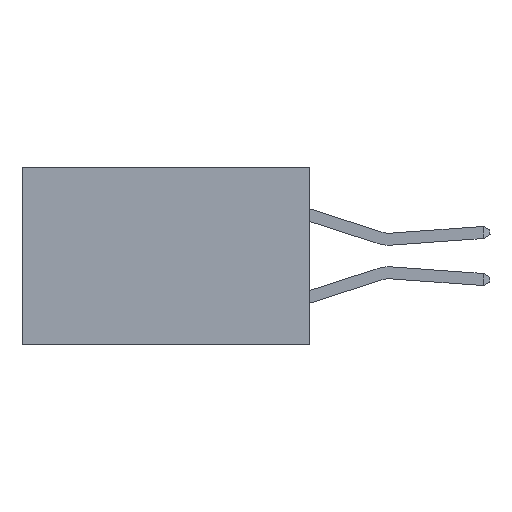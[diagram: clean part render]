
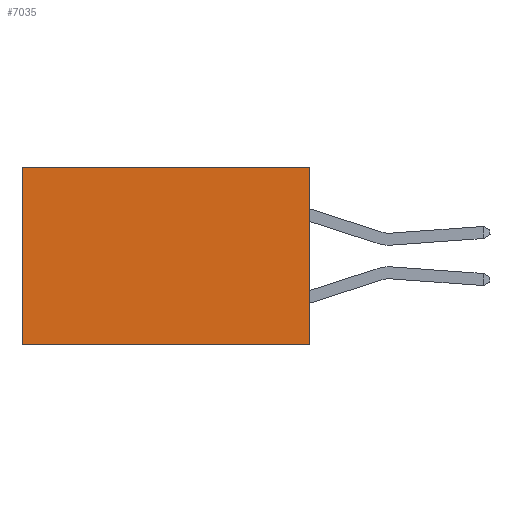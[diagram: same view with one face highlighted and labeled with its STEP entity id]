
A CAD part, left-side view. The second image highlights one B-rep face of the part: STEP entity #7035.
In plain terms, the highlighted planar face has unit normal (-1, 0, 0).
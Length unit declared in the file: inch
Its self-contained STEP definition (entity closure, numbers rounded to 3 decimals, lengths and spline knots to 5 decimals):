
#592 = CARTESIAN_POINT ( 'NONE',  ( 0.2615, 0., 0. ) ) ;
#673 = DIRECTION ( 'NONE',  ( 1., 0., 0. ) ) ;
#1024 = EDGE_CURVE ( 'NONE', #16479, #13670, #17530, .T. ) ;
#1749 = CARTESIAN_POINT ( 'NONE',  ( 0.2615, 0., -0.37 ) ) ;
#1981 = DIRECTION ( 'NONE',  ( 0., 0., -1. ) ) ;
#4610 = DIRECTION ( 'NONE',  ( 0., 0., -1. ) ) ;
#5098 = ORIENTED_EDGE ( 'NONE', *, *, #10494, .F. ) ;
#6005 = PLANE ( 'NONE',  #18022 ) ;
#7035 = ADVANCED_FACE ( 'NONE', ( #8070 ), #6005, .F. ) ;
#7647 = DIRECTION ( 'NONE',  ( 0., 1., 0. ) ) ;
#7846 = LINE ( 'NONE', #9695, #20229 ) ;
#8070 = FACE_OUTER_BOUND ( 'NONE', #13465, .T. ) ;
#8399 = CARTESIAN_POINT ( 'NONE',  ( 0.2615, 0.6, 0. ) ) ;
#9695 = CARTESIAN_POINT ( 'NONE',  ( 0.2615, 0., -0.37 ) ) ;
#9732 = ORIENTED_EDGE ( 'NONE', *, *, #21567, .T. ) ;
#9809 = CARTESIAN_POINT ( 'NONE',  ( 0.2615, 0., -0.37 ) ) ;
#10273 = CARTESIAN_POINT ( 'NONE',  ( 0.2615, 0., 0. ) ) ;
#10494 = EDGE_CURVE ( 'NONE', #13670, #15397, #7846, .T. ) ;
#11269 = EDGE_CURVE ( 'NONE', #16479, #18366, #18108, .T. ) ;
#13465 = EDGE_LOOP ( 'NONE', ( #9732, #5098, #20889, #18649 ) ) ;
#13670 = VERTEX_POINT ( 'NONE', #14851 ) ;
#13693 = VECTOR ( 'NONE', #1981, 39.37008 ) ;
#14851 = CARTESIAN_POINT ( 'NONE',  ( 0.2615, 0., -0.37 ) ) ;
#15397 = VERTEX_POINT ( 'NONE', #22271 ) ;
#15746 = VECTOR ( 'NONE', #4610, 39.37008 ) ;
#16479 = VERTEX_POINT ( 'NONE', #10273 ) ;
#16928 = CARTESIAN_POINT ( 'NONE',  ( 0.2615, 0.6, -0.37 ) ) ;
#16980 = VECTOR ( 'NONE', #7647, 39.37008 ) ;
#17530 = LINE ( 'NONE', #1749, #13693 ) ;
#18022 = AXIS2_PLACEMENT_3D ( 'NONE', #9809, #673, #20157 ) ;
#18108 = LINE ( 'NONE', #592, #16980 ) ;
#18366 = VERTEX_POINT ( 'NONE', #8399 ) ;
#18649 = ORIENTED_EDGE ( 'NONE', *, *, #11269, .T. ) ;
#20157 = DIRECTION ( 'NONE',  ( 0., 0., -1. ) ) ;
#20229 = VECTOR ( 'NONE', #21754, 39.37008 ) ;
#20889 = ORIENTED_EDGE ( 'NONE', *, *, #1024, .F. ) ;
#21567 = EDGE_CURVE ( 'NONE', #18366, #15397, #22322, .T. ) ;
#21754 = DIRECTION ( 'NONE',  ( 0., 1., 0. ) ) ;
#22271 = CARTESIAN_POINT ( 'NONE',  ( 0.2615, 0.6, -0.37 ) ) ;
#22322 = LINE ( 'NONE', #16928, #15746 ) ;
